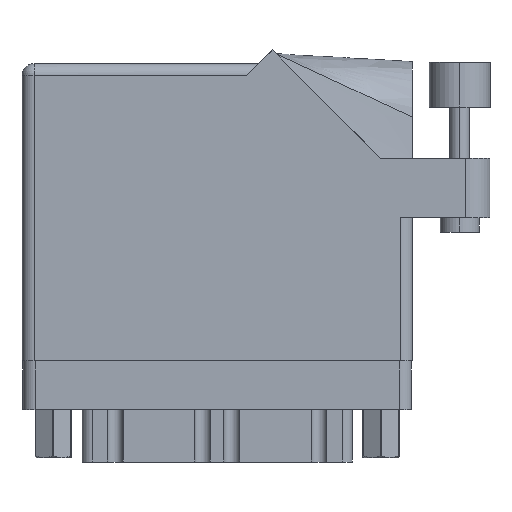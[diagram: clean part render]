
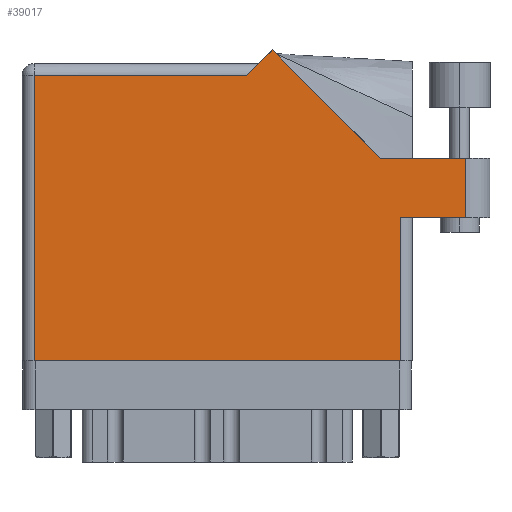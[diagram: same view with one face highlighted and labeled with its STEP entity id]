
A CAD part, front view. The second image highlights one B-rep face of the part: STEP entity #39017.
In plain terms, the highlighted face is planar.
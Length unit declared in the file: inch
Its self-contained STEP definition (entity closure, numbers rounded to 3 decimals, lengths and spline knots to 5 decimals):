
#164 = DIRECTION ( 'NONE',  ( -0.707, -0.707, 0. ) ) ;
#723 = LINE ( 'NONE', #22342, #41426 ) ;
#727 = VECTOR ( 'NONE', #46597, 39.37008 ) ;
#1021 = EDGE_CURVE ( 'NONE', #23415, #29377, #16420, .T. ) ;
#1283 = CARTESIAN_POINT ( 'NONE',  ( 0., 1.53, 0. ) ) ;
#1544 = DIRECTION ( 'NONE',  ( -1., 0., 0. ) ) ;
#1874 = ORIENTED_EDGE ( 'NONE', *, *, #18531, .T. ) ;
#1987 = ORIENTED_EDGE ( 'NONE', *, *, #40211, .T. ) ;
#2726 = EDGE_CURVE ( 'NONE', #46024, #23415, #13210, .T. ) ;
#3277 = CARTESIAN_POINT ( 'NONE',  ( 1.155, 1.468, 0. ) ) ;
#3914 = VERTEX_POINT ( 'NONE', #11310 ) ;
#4310 = AXIS2_PLACEMENT_3D ( 'NONE', #1283, #41366, #1544 ) ;
#4703 = ORIENTED_EDGE ( 'NONE', *, *, #23727, .T. ) ;
#4874 = CARTESIAN_POINT ( 'NONE',  ( 0.062, 0., 0. ) ) ;
#5712 = CARTESIAN_POINT ( 'NONE',  ( 1.84442, 1.044, 0. ) ) ;
#8289 = VECTOR ( 'NONE', #14296, 39.37008 ) ;
#8654 = ORIENTED_EDGE ( 'NONE', *, *, #2726, .T. ) ;
#9893 = LINE ( 'NONE', #17341, #727 ) ;
#10948 = EDGE_CURVE ( 'NONE', #25495, #47031, #32276, .T. ) ;
#10955 = DIRECTION ( 'NONE',  ( 1., 0., 0. ) ) ;
#11191 = DIRECTION ( 'NONE',  ( 0., 1., 0. ) ) ;
#11310 = CARTESIAN_POINT ( 'NONE',  ( 1.948, 0., 0. ) ) ;
#11414 = LINE ( 'NONE', #14568, #24314 ) ;
#12155 = VERTEX_POINT ( 'NONE', #5712 ) ;
#12205 = ORIENTED_EDGE ( 'NONE', *, *, #34450, .T. ) ;
#12571 = CARTESIAN_POINT ( 'NONE',  ( 0., 1.468, 0. ) ) ;
#13210 = LINE ( 'NONE', #22235, #35827 ) ;
#13338 = CARTESIAN_POINT ( 'NONE',  ( 2.285, 1.044, 0. ) ) ;
#14296 = DIRECTION ( 'NONE',  ( 1., 0., 0. ) ) ;
#14568 = CARTESIAN_POINT ( 'NONE',  ( 0., 0., 0. ) ) ;
#15026 = CARTESIAN_POINT ( 'NONE',  ( 1.28771, 1.60071, 0. ) ) ;
#15385 = DIRECTION ( 'NONE',  ( 0., 1., 0. ) ) ;
#15465 = VERTEX_POINT ( 'NONE', #13338 ) ;
#15518 = EDGE_LOOP ( 'NONE', ( #18530, #17292, #12205, #4703, #8654, #27242, #41643, #1987, #1874 ) ) ;
#16420 = LINE ( 'NONE', #12571, #37031 ) ;
#17173 = LINE ( 'NONE', #28165, #34904 ) ;
#17292 = ORIENTED_EDGE ( 'NONE', *, *, #38417, .T. ) ;
#17341 = CARTESIAN_POINT ( 'NONE',  ( 2.41, 1.044, 0. ) ) ;
#18447 = CARTESIAN_POINT ( 'NONE',  ( 0.062, 1.468, 0. ) ) ;
#18530 = ORIENTED_EDGE ( 'NONE', *, *, #10948, .T. ) ;
#18531 = EDGE_CURVE ( 'NONE', #3914, #25495, #723, .T. ) ;
#19536 = DIRECTION ( 'NONE',  ( 0., -1., 0. ) ) ;
#20932 = CARTESIAN_POINT ( 'NONE',  ( 0.062, 0., 0. ) ) ;
#22235 = CARTESIAN_POINT ( 'NONE',  ( 1.217, 1.53, 0. ) ) ;
#22342 = CARTESIAN_POINT ( 'NONE',  ( 1.948, 0.737, 0. ) ) ;
#23415 = VERTEX_POINT ( 'NONE', #3277 ) ;
#23727 = EDGE_CURVE ( 'NONE', #12155, #46024, #17173, .T. ) ;
#23873 = CARTESIAN_POINT ( 'NONE',  ( 1.948, 0.737, 0. ) ) ;
#24314 = VECTOR ( 'NONE', #10955, 39.37008 ) ;
#25495 = VERTEX_POINT ( 'NONE', #23873 ) ;
#26719 = FACE_OUTER_BOUND ( 'NONE', #15518, .T. ) ;
#27242 = ORIENTED_EDGE ( 'NONE', *, *, #1021, .T. ) ;
#27894 = DIRECTION ( 'NONE',  ( -1., 0., 0. ) ) ;
#28165 = CARTESIAN_POINT ( 'NONE',  ( 1.84442, 1.044, 0. ) ) ;
#29199 = CARTESIAN_POINT ( 'NONE',  ( 2.285, 1.044, 0. ) ) ;
#29377 = VERTEX_POINT ( 'NONE', #18447 ) ;
#29592 = VECTOR ( 'NONE', #19536, 39.37008 ) ;
#32276 = LINE ( 'NONE', #46927, #8289 ) ;
#34450 = EDGE_CURVE ( 'NONE', #15465, #12155, #9893, .T. ) ;
#34904 = VECTOR ( 'NONE', #46414, 39.37008 ) ;
#35827 = VECTOR ( 'NONE', #164, 39.37008 ) ;
#37031 = VECTOR ( 'NONE', #27894, 39.37008 ) ;
#37755 = LINE ( 'NONE', #4874, #29592 ) ;
#38417 = EDGE_CURVE ( 'NONE', #47031, #15465, #46970, .T. ) ;
#39017 = ADVANCED_FACE ( 'NONE', ( #26719 ), #40885, .F. ) ;
#39050 = EDGE_CURVE ( 'NONE', #29377, #45434, #37755, .T. ) ;
#40211 = EDGE_CURVE ( 'NONE', #45434, #3914, #11414, .T. ) ;
#40885 = PLANE ( 'NONE',  #4310 ) ;
#41366 = DIRECTION ( 'NONE',  ( 0., 0., -1. ) ) ;
#41426 = VECTOR ( 'NONE', #15385, 39.37008 ) ;
#41643 = ORIENTED_EDGE ( 'NONE', *, *, #39050, .T. ) ;
#44498 = CARTESIAN_POINT ( 'NONE',  ( 2.285, 0.737, 0. ) ) ;
#45434 = VERTEX_POINT ( 'NONE', #20932 ) ;
#46024 = VERTEX_POINT ( 'NONE', #15026 ) ;
#46414 = DIRECTION ( 'NONE',  ( -0.707, 0.707, 0. ) ) ;
#46432 = VECTOR ( 'NONE', #11191, 39.37008 ) ;
#46597 = DIRECTION ( 'NONE',  ( -1., 0., 0. ) ) ;
#46927 = CARTESIAN_POINT ( 'NONE',  ( 2.01, 0.737, 0. ) ) ;
#46970 = LINE ( 'NONE', #29199, #46432 ) ;
#47031 = VERTEX_POINT ( 'NONE', #44498 ) ;
